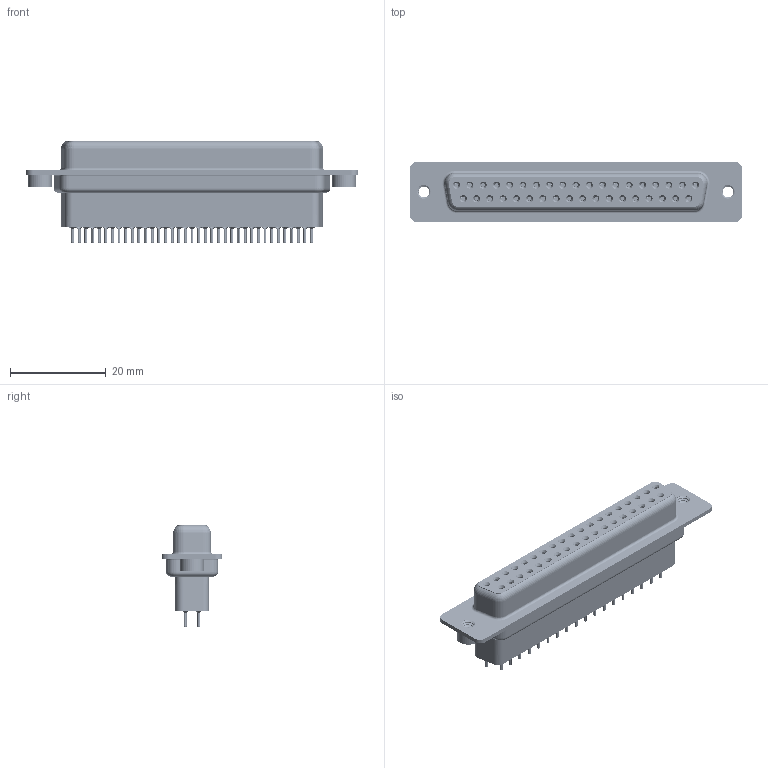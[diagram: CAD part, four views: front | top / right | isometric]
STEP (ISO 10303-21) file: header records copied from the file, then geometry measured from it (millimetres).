
FILE_DESCRIPTION (( 'STEP AP203' ), '1' );
FILE_NAME ('628-037-621-552.STEP', '2018-10-20T05:02:47', ( '' ), ( '' ), 'SwSTEP 2.0', 'SolidWorks 2016', '' );
FILE_SCHEMA (( 'CONFIG_CONTROL_DESIGN' ));
Length unit declared in the file: millimetre
Products named in the file (7): 628 Housing_37 HP; 628 Shell Front_37 Contacts; 628 Shell Rear_37 Contacts; 628 Contact Row 1_21H; 628 Contact Row 2_21H; 628 4-40 Threaded Rivet; 628-037-621-552
Assembly tree (42 placements, depth 2):
  628-037-621-552
    628 Housing_37 HP
    628 Shell Front_37 Contacts
    628 Shell Rear_37 Contacts
    628 Contact Row 1_21H  x19
    628 Contact Row 2_21H  x18
    628 4-40 Threaded Rivet  x2
Bounding box: 69.3 x 12.6 x 21.1 mm (x, y, z)
Volume: 7547.8 mm3; surface area: 16807.3 mm2
Topology: 42 solids, 42 shells, 4803 faces, 12312 edges, 7679 vertices
Faces by surface type: cylinder 1345, plane 1211, torus 940, bspline 746, cone 561
Entity records: 31857 total; most frequent: CARTESIAN_POINT 8469, DIRECTION 4858, ORIENTED_EDGE 4296, EDGE_CURVE 2148, AXIS2_PLACEMENT_3D 2046, VERTEX_POINT 1361, EDGE_LOOP 1127, CIRCLE 1124
